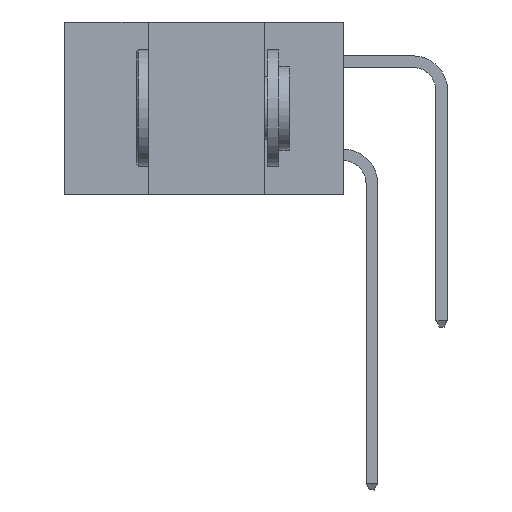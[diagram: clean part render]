
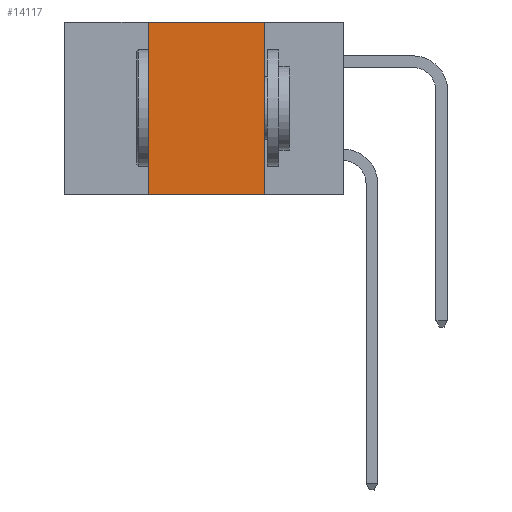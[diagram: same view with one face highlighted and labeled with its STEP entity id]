
A CAD part, left-side view. The second image highlights one B-rep face of the part: STEP entity #14117.
In plain terms, the highlighted planar face has unit normal (-1, 0, 0).
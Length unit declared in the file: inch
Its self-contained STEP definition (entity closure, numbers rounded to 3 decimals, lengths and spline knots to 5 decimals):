
#212 = ORIENTED_EDGE ( 'NONE', *, *, #17738, .F. ) ;
#386 = ORIENTED_EDGE ( 'NONE', *, *, #24532, .F. ) ;
#782 = VERTEX_POINT ( 'NONE', #11573 ) ;
#2789 = CARTESIAN_POINT ( 'NONE',  ( 0., 0.42, 0. ) ) ;
#3317 = CARTESIAN_POINT ( 'NONE',  ( 0., 0.17, 0. ) ) ;
#3474 = VERTEX_POINT ( 'NONE', #2789 ) ;
#4769 = CARTESIAN_POINT ( 'NONE',  ( 0., 0.6, 0. ) ) ;
#6733 = DIRECTION ( 'NONE',  ( 1., 0., 0. ) ) ;
#6975 = DIRECTION ( 'NONE',  ( 0., 0., 1. ) ) ;
#7023 = EDGE_LOOP ( 'NONE', ( #212, #14947, #386, #20043 ) ) ;
#7471 = VECTOR ( 'NONE', #22129, 39.37008 ) ;
#8990 = CARTESIAN_POINT ( 'NONE',  ( 0., 0.17, -0.37 ) ) ;
#9475 = VECTOR ( 'NONE', #22780, 39.37008 ) ;
#9480 = CARTESIAN_POINT ( 'NONE',  ( 0., 0.17, 0. ) ) ;
#11573 = CARTESIAN_POINT ( 'NONE',  ( 0., 0.42, -0.37 ) ) ;
#11726 = LINE ( 'NONE', #9480, #16248 ) ;
#12467 = PLANE ( 'NONE',  #16569 ) ;
#14117 = ADVANCED_FACE ( 'NONE', ( #19989 ), #12467, .F. ) ;
#14224 = VERTEX_POINT ( 'NONE', #8990 ) ;
#14371 = EDGE_CURVE ( 'NONE', #782, #14224, #14607, .T. ) ;
#14607 = LINE ( 'NONE', #24644, #9475 ) ;
#14780 = VECTOR ( 'NONE', #6975, 39.37008 ) ;
#14947 = ORIENTED_EDGE ( 'NONE', *, *, #17456, .F. ) ;
#15381 = LINE ( 'NONE', #20475, #14780 ) ;
#16248 = VECTOR ( 'NONE', #20966, 39.37008 ) ;
#16569 = AXIS2_PLACEMENT_3D ( 'NONE', #4769, #6733, #20231 ) ;
#17456 = EDGE_CURVE ( 'NONE', #3474, #20184, #17729, .T. ) ;
#17729 = LINE ( 'NONE', #22045, #7471 ) ;
#17738 = EDGE_CURVE ( 'NONE', #20184, #14224, #11726, .T. ) ;
#19989 = FACE_OUTER_BOUND ( 'NONE', #7023, .T. ) ;
#20043 = ORIENTED_EDGE ( 'NONE', *, *, #14371, .T. ) ;
#20184 = VERTEX_POINT ( 'NONE', #3317 ) ;
#20231 = DIRECTION ( 'NONE',  ( 0., 0., -1. ) ) ;
#20475 = CARTESIAN_POINT ( 'NONE',  ( 0., 0.42, 0. ) ) ;
#20966 = DIRECTION ( 'NONE',  ( 0., 0., -1. ) ) ;
#22045 = CARTESIAN_POINT ( 'NONE',  ( 0., 0.6, 0. ) ) ;
#22129 = DIRECTION ( 'NONE',  ( 0., -1., 0. ) ) ;
#22780 = DIRECTION ( 'NONE',  ( 0., -1., 0. ) ) ;
#24532 = EDGE_CURVE ( 'NONE', #782, #3474, #15381, .T. ) ;
#24644 = CARTESIAN_POINT ( 'NONE',  ( 0., 0.6, -0.37 ) ) ;
